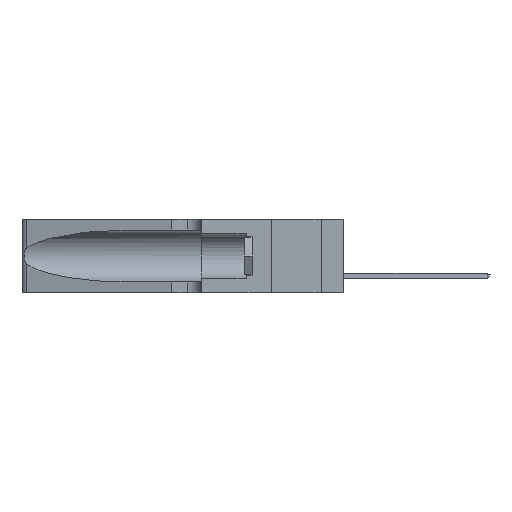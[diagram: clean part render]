
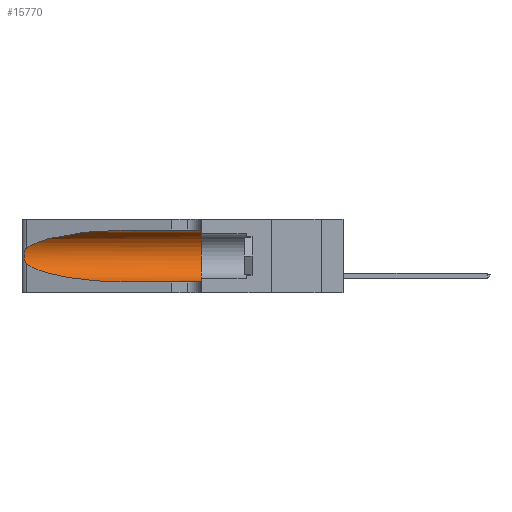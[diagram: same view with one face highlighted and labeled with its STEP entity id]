
A CAD part, left-side view. The second image highlights one B-rep face of the part: STEP entity #15770.
In plain terms, the highlighted cylindrical face has radius 3.308 mm (diameter 6.617 mm), a partial arc.
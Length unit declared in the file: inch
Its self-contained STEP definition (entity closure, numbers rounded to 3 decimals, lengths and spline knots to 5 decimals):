
#800 = CARTESIAN_POINT ( 'NONE',  ( 0.1305, 0.72297, 0.31525 ) ) ;
#2071 = VERTEX_POINT ( 'NONE', #14736 ) ;
#4950 = VERTEX_POINT ( 'NONE', #31954 ) ;
#5450 = ORIENTED_EDGE ( 'NONE', *, *, #26012, .T. ) ;
#5647 = CARTESIAN_POINT ( 'NONE',  ( 0.26075, 1.23896, 0.178 ) ) ;
#6631 = CARTESIAN_POINT ( 'NONE',  ( 0.1305, 0.72297, 0.31525 ) ) ;
#6803 = CARTESIAN_POINT ( 'NONE',  ( 0.1305, 1.61858, 0.31525 ) ) ;
#6811 = EDGE_CURVE ( 'NONE', #4950, #25481, #32935, .T. ) ;
#6827 = CARTESIAN_POINT ( 'NONE',  ( 0.1305, 0.72297, 0.05475 ) ) ;
#7288 = CARTESIAN_POINT ( 'NONE',  ( 0.25487, 1.22718, 0.22369 ) ) ;
#8165 = CARTESIAN_POINT ( 'NONE',  ( 0.25555, 1.22993, 0.14849 ) ) ;
#8852 = CARTESIAN_POINT ( 'NONE',  ( 0.25487, 1.22718, 0.14631 ) ) ;
#11091 = LINE ( 'NONE', #18521, #11985 ) ;
#11138 = AXIS2_PLACEMENT_3D ( 'NONE', #25046, #14164, #13956 ) ;
#11790 = CARTESIAN_POINT ( 'NONE',  ( 0.18966, 0.96281, 0.31525 ) ) ;
#11985 = VECTOR ( 'NONE', #33586, 39.37008 ) ;
#12712 = CARTESIAN_POINT ( 'NONE',  ( 0.18966, 0.96281, 0.05475 ) ) ;
#13314 = CARTESIAN_POINT ( 'NONE',  ( 0.1305, 0.72297, 0.05475 ) ) ;
#13956 = DIRECTION ( 'NONE',  ( 0., 0., 1. ) ) ;
#14164 = DIRECTION ( 'NONE',  ( 0., 1., 0. ) ) ;
#14292 = CARTESIAN_POINT ( 'NONE',  ( 0.26017, 1.23833, 0.17102 ) ) ;
#14736 = CARTESIAN_POINT ( 'NONE',  ( 0.1305, 0.35, 0.05475 ) ) ;
#15770 = ADVANCED_FACE ( 'NONE', ( #34449 ), #24611, .F. ) ;
#15899 = CARTESIAN_POINT ( 'NONE',  ( 0.1305, 0.35, 0.31525 ) ) ;
#15926 = ORIENTED_EDGE ( 'NONE', *, *, #17129, .F. ) ;
#17129 = EDGE_CURVE ( 'NONE', #23786, #2071, #19403, .T. ) ;
#17183 = EDGE_CURVE ( 'NONE', #35439, #4950, #20658, .T. ) ;
#17990 =( BOUNDED_CURVE ( )  B_SPLINE_CURVE ( 3, ( #34674, #20539, #12712, #6827 ),
 .UNSPECIFIED., .F., .F. ) 
 B_SPLINE_CURVE_WITH_KNOTS ( ( 4, 4 ),
 ( 3.44316, 4.71239 ),
 .UNSPECIFIED. ) 
 CURVE ( )  GEOMETRIC_REPRESENTATION_ITEM ( )  RATIONAL_B_SPLINE_CURVE ( ( 1., 0.87, 0.87, 1. ) ) 
 REPRESENTATION_ITEM ( '' )  );
#18521 = CARTESIAN_POINT ( 'NONE',  ( 0.1305, 1.61858, 0.05475 ) ) ;
#18691 = VERTEX_POINT ( 'NONE', #13314 ) ;
#19082 = DIRECTION ( 'NONE',  ( 0., 0., -1. ) ) ;
#19351 = CARTESIAN_POINT ( 'NONE',  ( 0.25856, 1.23593, 0.16098 ) ) ;
#19403 = CIRCLE ( 'NONE', #11138, 0.13025 ) ;
#20093 = CARTESIAN_POINT ( 'NONE',  ( 0.25639, 1.23184, 0.21858 ) ) ;
#20205 = CARTESIAN_POINT ( 'NONE',  ( 0.25487, 1.22718, 0.22369 ) ) ;
#20539 = CARTESIAN_POINT ( 'NONE',  ( 0.2373, 1.15595, 0.08982 ) ) ;
#20595 = CARTESIAN_POINT ( 'NONE',  ( 0.25639, 1.23186, 0.15144 ) ) ;
#20658 =( BOUNDED_CURVE ( )  B_SPLINE_CURVE ( 3, ( #6631, #11790, #25909, #20205 ),
 .UNSPECIFIED., .F., .F. ) 
 B_SPLINE_CURVE_WITH_KNOTS ( ( 4, 4 ),
 ( 1.5708, 2.84003 ),
 .UNSPECIFIED. ) 
 CURVE ( )  GEOMETRIC_REPRESENTATION_ITEM ( )  RATIONAL_B_SPLINE_CURVE ( ( 1., 0.87, 0.87, 1. ) ) 
 REPRESENTATION_ITEM ( '' )  );
#22021 = LINE ( 'NONE', #6803, #28491 ) ;
#22075 = ORIENTED_EDGE ( 'NONE', *, *, #6811, .T. ) ;
#22356 = CARTESIAN_POINT ( 'NONE',  ( 0.25789, 1.23486, 0.15765 ) ) ;
#22609 = ORIENTED_EDGE ( 'NONE', *, *, #24482, .F. ) ;
#22953 = CARTESIAN_POINT ( 'NONE',  ( 0.26018, 1.23835, 0.19895 ) ) ;
#23786 = VERTEX_POINT ( 'NONE', #15899 ) ;
#24482 = EDGE_CURVE ( 'NONE', #35439, #23786, #22021, .T. ) ;
#24611 = CYLINDRICAL_SURFACE ( 'NONE', #26029, 0.13025 ) ;
#25046 = CARTESIAN_POINT ( 'NONE',  ( 0.1305, 0.35, 0.185 ) ) ;
#25481 = VERTEX_POINT ( 'NONE', #30723 ) ;
#25909 = CARTESIAN_POINT ( 'NONE',  ( 0.2373, 1.15595, 0.28018 ) ) ;
#26012 = EDGE_CURVE ( 'NONE', #18691, #2071, #11091, .T. ) ;
#26029 = AXIS2_PLACEMENT_3D ( 'NONE', #29228, #35420, #19082 ) ;
#26079 = DIRECTION ( 'NONE',  ( 0., -1., 0. ) ) ;
#28491 = VECTOR ( 'NONE', #26079, 39.37008 ) ;
#29081 = EDGE_LOOP ( 'NONE', ( #32074, #22075, #32557, #5450, #15926, #22609 ) ) ;
#29109 = EDGE_CURVE ( 'NONE', #25481, #18691, #17990, .T. ) ;
#29228 = CARTESIAN_POINT ( 'NONE',  ( 0.1305, 1.61858, 0.185 ) ) ;
#30723 = CARTESIAN_POINT ( 'NONE',  ( 0.25487, 1.22718, 0.14631 ) ) ;
#31953 = CARTESIAN_POINT ( 'NONE',  ( 0.25787, 1.23484, 0.2124 ) ) ;
#31954 = CARTESIAN_POINT ( 'NONE',  ( 0.25487, 1.22718, 0.22369 ) ) ;
#32074 = ORIENTED_EDGE ( 'NONE', *, *, #17183, .T. ) ;
#32557 = ORIENTED_EDGE ( 'NONE', *, *, #29109, .T. ) ;
#32935 = B_SPLINE_CURVE_WITH_KNOTS ( 'NONE', 3,
 ( #7288, #34901, #20093, #31953, #35323, #22953, #33352, #5647, #14292, #19351, #22356, #20595, #8165, #8852 ),
 .UNSPECIFIED., .F., .F.,
 ( 4, 2, 2, 2, 2, 2, 4 ),
 ( 0., 0.00027, 0.00053, 0.00107, 0.0016, 0.00187, 0.00214 ),
 .UNSPECIFIED. ) ;
#33352 = CARTESIAN_POINT ( 'NONE',  ( 0.26075, 1.23896, 0.19203 ) ) ;
#33586 = DIRECTION ( 'NONE',  ( 0., -1., 0. ) ) ;
#34449 = FACE_OUTER_BOUND ( 'NONE', #29081, .T. ) ;
#34674 = CARTESIAN_POINT ( 'NONE',  ( 0.25487, 1.22718, 0.14631 ) ) ;
#34901 = CARTESIAN_POINT ( 'NONE',  ( 0.25555, 1.22994, 0.2215 ) ) ;
#35323 = CARTESIAN_POINT ( 'NONE',  ( 0.25854, 1.2359, 0.20912 ) ) ;
#35420 = DIRECTION ( 'NONE',  ( 0., -1., 0. ) ) ;
#35439 = VERTEX_POINT ( 'NONE', #800 ) ;
